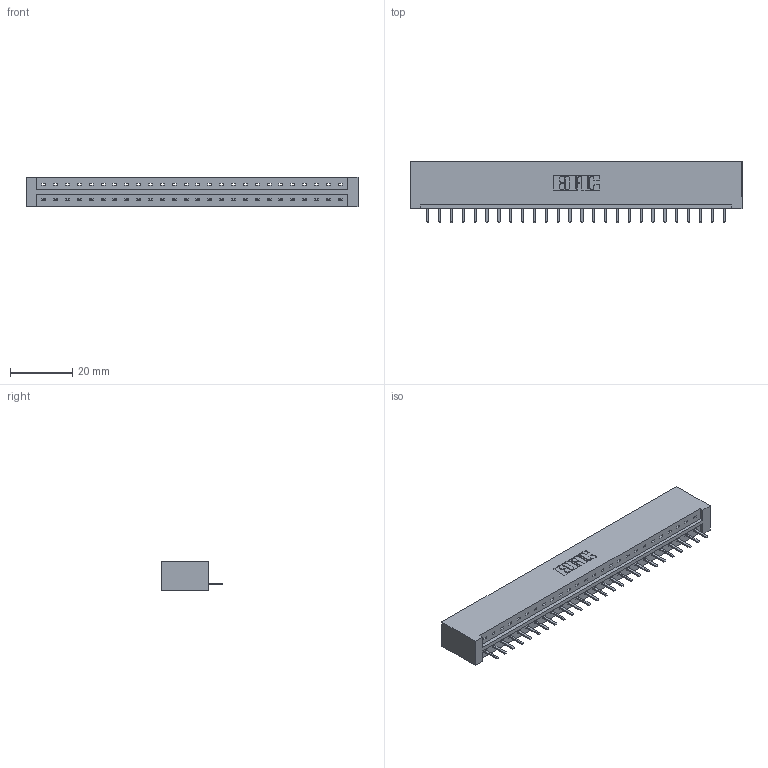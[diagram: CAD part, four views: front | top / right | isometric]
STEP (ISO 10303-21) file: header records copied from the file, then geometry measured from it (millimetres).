
FILE_DESCRIPTION (( 'STEP AP203' ), '1' );
FILE_NAME ('379-026-520-101.STEP', '2020-02-26T15:24:29', ( '' ), ( '' ), 'SwSTEP 2.0', 'SolidWorks 2016', '' );
FILE_SCHEMA (( 'CONFIG_CONTROL_DESIGN' ));
Length unit declared in the file: inch
Products named in the file (3): 345-292-001_345-293-120; 379-026-520-101; 379 Part_Lugless
Assembly tree (27 placements, depth 2):
  379-026-520-101
    379 Part_Lugless
    345-292-001_345-293-120  x26
Bounding box: 106.68 x 19.68 x 9.53 mm (x, y, z)
Volume: 11662.2 mm3; surface area: 11548.8 mm2
Topology: 27 solids, 27 shells, 1718 faces, 5071 edges, 3310 vertices
Faces by surface type: plane 1210, cylinder 508
Entity records: 17801 total; most frequent: CARTESIAN_POINT 3092, ORIENTED_EDGE 3042, DIRECTION 2621, EDGE_CURVE 1521, VECTOR 1397, LINE 1397, VERTEX_POINT 1010, AXIS2_PLACEMENT_3D 612
